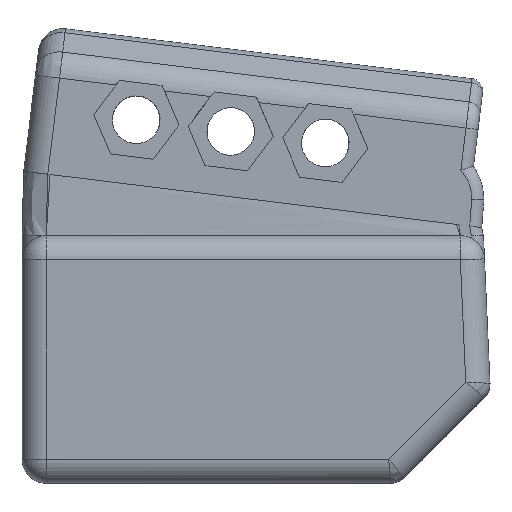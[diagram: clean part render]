
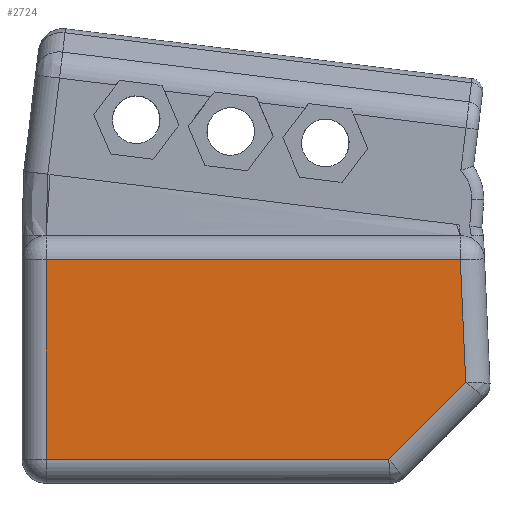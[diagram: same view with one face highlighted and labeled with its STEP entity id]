
A CAD part, left-side view. The second image highlights one B-rep face of the part: STEP entity #2724.
In plain terms, the highlighted planar face has unit normal (-1, 0, 0).
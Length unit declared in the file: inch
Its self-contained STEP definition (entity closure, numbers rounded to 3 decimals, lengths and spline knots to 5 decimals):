
#66=PLANE('',#2954);
#230=FACE_OUTER_BOUND('',#394,.T.);
#394=EDGE_LOOP('',(#2029,#2030,#2031,#2032,#2033));
#717=LINE('',#5286,#944);
#722=LINE('',#5326,#949);
#725=LINE('',#5343,#952);
#728=LINE('',#5353,#955);
#729=LINE('',#5354,#956);
#944=VECTOR('',#3351,0.3937);
#949=VECTOR('',#3378,0.3937);
#952=VECTOR('',#3401,0.3937);
#955=VECTOR('',#3414,0.3937);
#956=VECTOR('',#3415,0.3937);
#1211=VERTEX_POINT('',#5283);
#1212=VERTEX_POINT('',#5285);
#1220=VERTEX_POINT('',#5324);
#1224=VERTEX_POINT('',#5341);
#1226=VERTEX_POINT('',#5352);
#1506=EDGE_CURVE('',#1211,#1212,#717,.T.);
#1520=EDGE_CURVE('',#1220,#1211,#722,.T.);
#1530=EDGE_CURVE('',#1224,#1220,#725,.T.);
#1533=EDGE_CURVE('',#1226,#1224,#728,.T.);
#1534=EDGE_CURVE('',#1212,#1226,#729,.T.);
#2029=ORIENTED_EDGE('',*,*,#1520,.F.);
#2030=ORIENTED_EDGE('',*,*,#1530,.F.);
#2031=ORIENTED_EDGE('',*,*,#1533,.F.);
#2032=ORIENTED_EDGE('',*,*,#1534,.F.);
#2033=ORIENTED_EDGE('',*,*,#1506,.F.);
#2724=ADVANCED_FACE('',(#230),#66,.F.);
#2954=AXIS2_PLACEMENT_3D('',#5351,#3412,#3413);
#3351=DIRECTION('',(0.,-0.044,-0.999));
#3378=DIRECTION('',(0.,-1.,0.));
#3401=DIRECTION('',(0.,0.,1.));
#3412=DIRECTION('center_axis',(1.,0.,0.));
#3413=DIRECTION('ref_axis',(0.,0.,1.));
#3414=DIRECTION('',(0.,1.,0.));
#3415=DIRECTION('',(0.,0.707,-0.707));
#5283=CARTESIAN_POINT('',(-0.80617,-0.65698,0.54503));
#5285=CARTESIAN_POINT('',(-0.80617,-0.67949,0.03978));
#5286=CARTESIAN_POINT('',(-0.80617,-0.50886,3.87113));
#5324=CARTESIAN_POINT('',(-0.80617,1.055,0.54503));
#5326=CARTESIAN_POINT('',(-0.80617,1.24673,0.54503));
#5341=CARTESIAN_POINT('',(-0.80617,1.055,-0.27859));
#5343=CARTESIAN_POINT('',(-0.80617,1.055,4.95113));
#5351=CARTESIAN_POINT('Origin',(-0.80617,1.155,-0.93963));
#5352=CARTESIAN_POINT('',(-0.80617,-0.36112,-0.27859));
#5353=CARTESIAN_POINT('',(-0.80617,0.78732,-0.27859));
#5354=CARTESIAN_POINT('',(-0.80617,0.04235,-0.68206));
